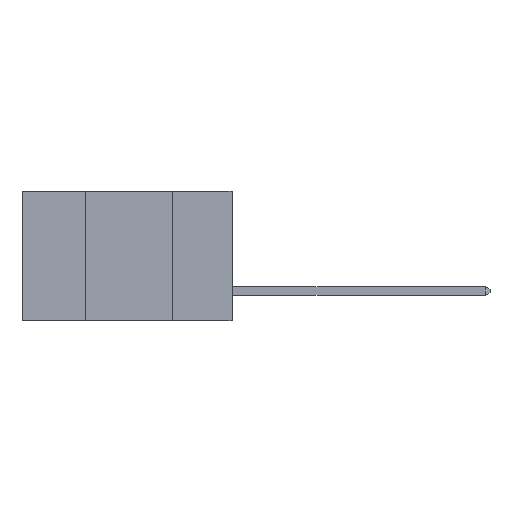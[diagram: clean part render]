
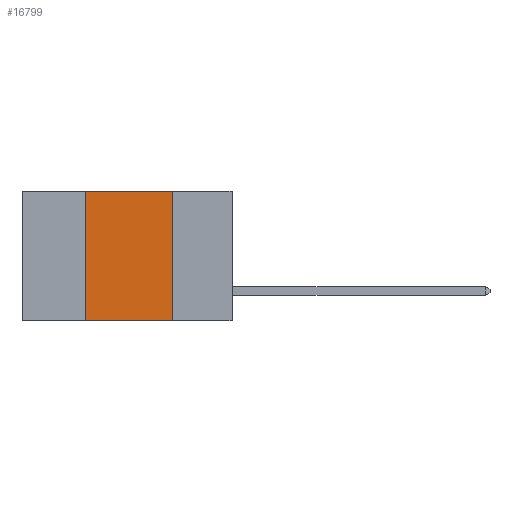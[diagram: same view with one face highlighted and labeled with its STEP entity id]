
A CAD part, left-side view. The second image highlights one B-rep face of the part: STEP entity #16799.
In plain terms, the highlighted planar face has unit normal (-1, 0, 0).
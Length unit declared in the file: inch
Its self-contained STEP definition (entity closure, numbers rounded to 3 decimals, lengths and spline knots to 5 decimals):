
#102 = VERTEX_POINT ( 'NONE', #2895 ) ;
#142 = ORIENTED_EDGE ( 'NONE', *, *, #20005, .T. ) ;
#479 = CARTESIAN_POINT ( 'NONE',  ( 0., 0.6, 0. ) ) ;
#1000 = CARTESIAN_POINT ( 'NONE',  ( 0., 0.42, 0. ) ) ;
#2895 = CARTESIAN_POINT ( 'NONE',  ( 0., 0.42, -0.37 ) ) ;
#3180 = ORIENTED_EDGE ( 'NONE', *, *, #22473, .F. ) ;
#3181 = DIRECTION ( 'NONE',  ( 0., 0., -1. ) ) ;
#4002 = VECTOR ( 'NONE', #24146, 39.37008 ) ;
#4955 = CARTESIAN_POINT ( 'NONE',  ( 0., 0.17, 0. ) ) ;
#4972 = LINE ( 'NONE', #35684, #4002 ) ;
#5686 = VECTOR ( 'NONE', #3181, 39.37008 ) ;
#7836 = LINE ( 'NONE', #479, #23697 ) ;
#11598 = AXIS2_PLACEMENT_3D ( 'NONE', #12456, #33085, #15481 ) ;
#11811 = ORIENTED_EDGE ( 'NONE', *, *, #12982, .F. ) ;
#12456 = CARTESIAN_POINT ( 'NONE',  ( 0., 0.6, 0. ) ) ;
#12982 = EDGE_CURVE ( 'NONE', #17803, #15917, #7836, .T. ) ;
#15059 = EDGE_CURVE ( 'NONE', #102, #17803, #17516, .T. ) ;
#15356 = PLANE ( 'NONE',  #11598 ) ;
#15481 = DIRECTION ( 'NONE',  ( 0., 0., -1. ) ) ;
#15917 = VERTEX_POINT ( 'NONE', #4955 ) ;
#16799 = ADVANCED_FACE ( 'NONE', ( #24808 ), #15356, .F. ) ;
#17516 = LINE ( 'NONE', #1000, #24422 ) ;
#17803 = VERTEX_POINT ( 'NONE', #19674 ) ;
#18215 = CARTESIAN_POINT ( 'NONE',  ( 0., 0.17, 0. ) ) ;
#19674 = CARTESIAN_POINT ( 'NONE',  ( 0., 0.42, 0. ) ) ;
#20005 = EDGE_CURVE ( 'NONE', #102, #30177, #4972, .T. ) ;
#21564 = DIRECTION ( 'NONE',  ( 0., -1., 0. ) ) ;
#21802 = ORIENTED_EDGE ( 'NONE', *, *, #15059, .F. ) ;
#22473 = EDGE_CURVE ( 'NONE', #15917, #30177, #37236, .T. ) ;
#23697 = VECTOR ( 'NONE', #21564, 39.37008 ) ;
#24146 = DIRECTION ( 'NONE',  ( 0., -1., 0. ) ) ;
#24422 = VECTOR ( 'NONE', #33739, 39.37008 ) ;
#24808 = FACE_OUTER_BOUND ( 'NONE', #31674, .T. ) ;
#28864 = CARTESIAN_POINT ( 'NONE',  ( 0., 0.17, -0.37 ) ) ;
#30177 = VERTEX_POINT ( 'NONE', #28864 ) ;
#31674 = EDGE_LOOP ( 'NONE', ( #3180, #11811, #21802, #142 ) ) ;
#33085 = DIRECTION ( 'NONE',  ( 1., 0., 0. ) ) ;
#33739 = DIRECTION ( 'NONE',  ( 0., 0., 1. ) ) ;
#35684 = CARTESIAN_POINT ( 'NONE',  ( 0., 0.6, -0.37 ) ) ;
#37236 = LINE ( 'NONE', #18215, #5686 ) ;
